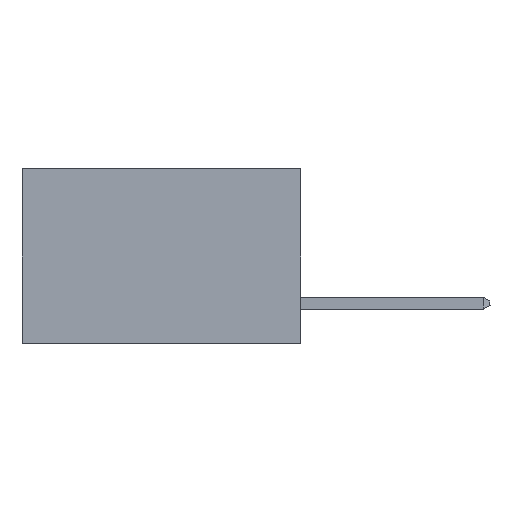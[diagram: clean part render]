
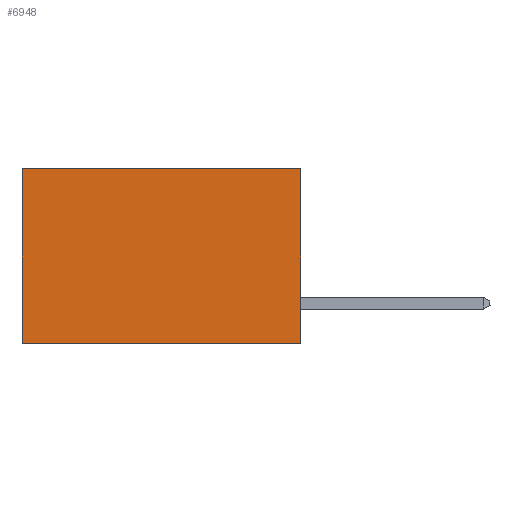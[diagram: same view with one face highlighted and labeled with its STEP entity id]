
A CAD part, left-side view. The second image highlights one B-rep face of the part: STEP entity #6948.
In plain terms, the highlighted planar face has unit normal (-1, 0, 0).
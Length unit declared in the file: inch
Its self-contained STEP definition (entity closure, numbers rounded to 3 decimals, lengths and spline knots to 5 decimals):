
#143 = LINE ( 'NONE', #10244, #791 ) ;
#357 = CARTESIAN_POINT ( 'NONE',  ( 0.277, 0.59, -0.37 ) ) ;
#791 = VECTOR ( 'NONE', #10929, 39.37008 ) ;
#1504 = VERTEX_POINT ( 'NONE', #7042 ) ;
#2487 = ORIENTED_EDGE ( 'NONE', *, *, #2846, .T. ) ;
#2661 = EDGE_CURVE ( 'NONE', #1504, #22711, #14229, .T. ) ;
#2846 = EDGE_CURVE ( 'NONE', #1504, #18332, #143, .T. ) ;
#3841 = EDGE_LOOP ( 'NONE', ( #8914, #10069, #15164, #2487 ) ) ;
#4617 = LINE ( 'NONE', #9448, #6971 ) ;
#6948 = ADVANCED_FACE ( 'NONE', ( #7299 ), #13648, .F. ) ;
#6971 = VECTOR ( 'NONE', #22106, 39.37008 ) ;
#7042 = CARTESIAN_POINT ( 'NONE',  ( 0.277, 0., 0. ) ) ;
#7299 = FACE_OUTER_BOUND ( 'NONE', #3841, .T. ) ;
#8914 = ORIENTED_EDGE ( 'NONE', *, *, #15034, .T. ) ;
#8921 = EDGE_CURVE ( 'NONE', #22711, #14149, #4617, .T. ) ;
#9408 = VECTOR ( 'NONE', #17869, 39.37008 ) ;
#9448 = CARTESIAN_POINT ( 'NONE',  ( 0.277, 0., -0.37 ) ) ;
#10069 = ORIENTED_EDGE ( 'NONE', *, *, #8921, .F. ) ;
#10244 = CARTESIAN_POINT ( 'NONE',  ( 0.277, 0., 0. ) ) ;
#10299 = AXIS2_PLACEMENT_3D ( 'NONE', #13490, #13423, #13416 ) ;
#10929 = DIRECTION ( 'NONE',  ( 0., 1., 0. ) ) ;
#11265 = DIRECTION ( 'NONE',  ( 0., 0., -1. ) ) ;
#13416 = DIRECTION ( 'NONE',  ( 0., 0., -1. ) ) ;
#13423 = DIRECTION ( 'NONE',  ( 1., 0., 0. ) ) ;
#13490 = CARTESIAN_POINT ( 'NONE',  ( 0.277, 0., -0.37 ) ) ;
#13648 = PLANE ( 'NONE',  #10299 ) ;
#14149 = VERTEX_POINT ( 'NONE', #357 ) ;
#14229 = LINE ( 'NONE', #18844, #9408 ) ;
#14551 = LINE ( 'NONE', #20281, #18799 ) ;
#15034 = EDGE_CURVE ( 'NONE', #18332, #14149, #14551, .T. ) ;
#15164 = ORIENTED_EDGE ( 'NONE', *, *, #2661, .F. ) ;
#17720 = CARTESIAN_POINT ( 'NONE',  ( 0.277, 0.59, 0. ) ) ;
#17869 = DIRECTION ( 'NONE',  ( 0., 0., -1. ) ) ;
#18131 = CARTESIAN_POINT ( 'NONE',  ( 0.277, 0., -0.37 ) ) ;
#18332 = VERTEX_POINT ( 'NONE', #17720 ) ;
#18799 = VECTOR ( 'NONE', #11265, 39.37008 ) ;
#18844 = CARTESIAN_POINT ( 'NONE',  ( 0.277, 0., -0.37 ) ) ;
#20281 = CARTESIAN_POINT ( 'NONE',  ( 0.277, 0.59, -0.37 ) ) ;
#22106 = DIRECTION ( 'NONE',  ( 0., 1., 0. ) ) ;
#22711 = VERTEX_POINT ( 'NONE', #18131 ) ;
